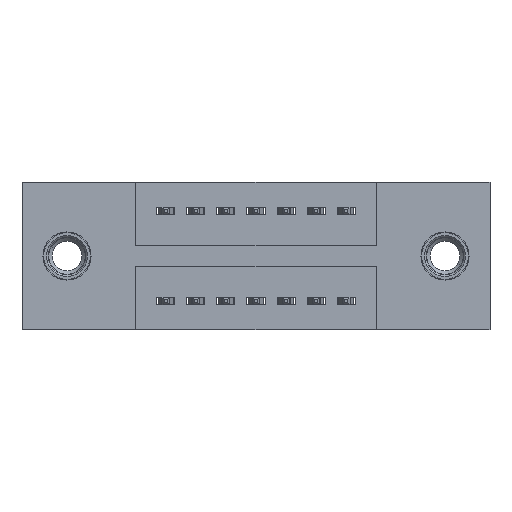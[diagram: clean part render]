
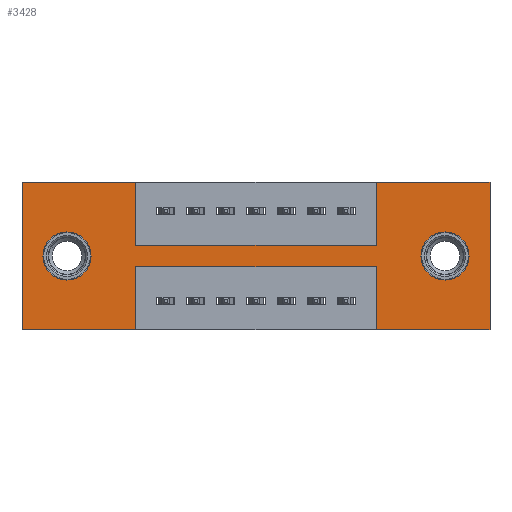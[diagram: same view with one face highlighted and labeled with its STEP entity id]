
A CAD part, front view. The second image highlights one B-rep face of the part: STEP entity #3428.
In plain terms, the highlighted planar face has unit normal (0, -1, 0).
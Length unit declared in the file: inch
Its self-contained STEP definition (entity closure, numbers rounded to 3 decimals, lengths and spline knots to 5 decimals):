
#21 = CARTESIAN_POINT ( 'NONE',  ( 1.1775, 0., -0.21 ) ) ;
#37 = LINE ( 'NONE', #5412, #4712 ) ;
#137 = AXIS2_PLACEMENT_3D ( 'NONE', #9034, #8138, #1855 ) ;
#304 = CARTESIAN_POINT ( 'NONE',  ( 1.4055, 0., -0.325 ) ) ;
#337 = EDGE_CURVE ( 'NONE', #5619, #1112, #37, .T. ) ;
#703 = ORIENTED_EDGE ( 'NONE', *, *, #7558, .T. ) ;
#708 = EDGE_CURVE ( 'NONE', #3977, #9456, #5096, .T. ) ;
#747 = ORIENTED_EDGE ( 'NONE', *, *, #9672, .T. ) ;
#772 = DIRECTION ( 'NONE',  ( -1., 0., 0. ) ) ;
#847 = VERTEX_POINT ( 'NONE', #9888 ) ;
#853 = CARTESIAN_POINT ( 'NONE',  ( 0.1495, 0., -0.245 ) ) ;
#908 = ORIENTED_EDGE ( 'NONE', *, *, #8822, .F. ) ;
#981 = ORIENTED_EDGE ( 'NONE', *, *, #4934, .F. ) ;
#989 = EDGE_CURVE ( 'NONE', #1058, #3947, #5598, .T. ) ;
#1058 = VERTEX_POINT ( 'NONE', #7208 ) ;
#1087 = EDGE_CURVE ( 'NONE', #4952, #6280, #4231, .T. ) ;
#1112 = VERTEX_POINT ( 'NONE', #4107 ) ;
#1210 = CARTESIAN_POINT ( 'NONE',  ( 0.3775, 0., -0.28 ) ) ;
#1282 = DIRECTION ( 'NONE',  ( 0., 0., -1. ) ) ;
#1493 = ORIENTED_EDGE ( 'NONE', *, *, #1875, .F. ) ;
#1513 = DIRECTION ( 'NONE',  ( 0., 0., -1. ) ) ;
#1626 = CARTESIAN_POINT ( 'NONE',  ( 1.1775, 0., -0.49 ) ) ;
#1719 = VECTOR ( 'NONE', #6772, 39.37008 ) ;
#1808 = DIRECTION ( 'NONE',  ( 1., 0., 0. ) ) ;
#1855 = DIRECTION ( 'NONE',  ( 0., 0., -1. ) ) ;
#1875 = EDGE_CURVE ( 'NONE', #847, #4952, #6077, .T. ) ;
#1997 = DIRECTION ( 'NONE',  ( 0., 1., 0. ) ) ;
#2097 = CARTESIAN_POINT ( 'NONE',  ( 1.1775, 0., -0.21 ) ) ;
#2109 = VECTOR ( 'NONE', #772, 39.37008 ) ;
#2134 = CARTESIAN_POINT ( 'NONE',  ( 1.4055, 0., -0.245 ) ) ;
#2318 = LINE ( 'NONE', #7312, #7439 ) ;
#2437 = DIRECTION ( 'NONE',  ( -1., 0., 0. ) ) ;
#2461 = EDGE_CURVE ( 'NONE', #9456, #7937, #5810, .T. ) ;
#2532 = DIRECTION ( 'NONE',  ( 0., 0., 1. ) ) ;
#2781 = DIRECTION ( 'NONE',  ( 0., 0., 1. ) ) ;
#2905 = CARTESIAN_POINT ( 'NONE',  ( 0.1495, 0., -0.325 ) ) ;
#3004 = VERTEX_POINT ( 'NONE', #3969 ) ;
#3428 = ADVANCED_FACE ( 'NONE', ( #10253, #8640, #8649 ), #7069, .T. ) ;
#3559 = LINE ( 'NONE', #6745, #9177 ) ;
#3593 = VERTEX_POINT ( 'NONE', #5746 ) ;
#3770 = AXIS2_PLACEMENT_3D ( 'NONE', #853, #4056, #7134 ) ;
#3772 = CARTESIAN_POINT ( 'NONE',  ( 0., 0., 0. ) ) ;
#3821 = DIRECTION ( 'NONE',  ( 0., 0., -1. ) ) ;
#3862 = EDGE_LOOP ( 'NONE', ( #747, #5677 ) ) ;
#3917 = ORIENTED_EDGE ( 'NONE', *, *, #2461, .F. ) ;
#3918 = VECTOR ( 'NONE', #4582, 39.37008 ) ;
#3947 = VERTEX_POINT ( 'NONE', #2905 ) ;
#3969 = CARTESIAN_POINT ( 'NONE',  ( 1.1775, 0., 0. ) ) ;
#3977 = VERTEX_POINT ( 'NONE', #5399 ) ;
#4003 = EDGE_CURVE ( 'NONE', #3004, #847, #8522, .T. ) ;
#4014 = ORIENTED_EDGE ( 'NONE', *, *, #8997, .F. ) ;
#4056 = DIRECTION ( 'NONE',  ( 0., 1., 0. ) ) ;
#4107 = CARTESIAN_POINT ( 'NONE',  ( 0.3775, 0., -0.21 ) ) ;
#4170 = AXIS2_PLACEMENT_3D ( 'NONE', #2134, #7713, #1282 ) ;
#4183 = DIRECTION ( 'NONE',  ( -1., 0., 0. ) ) ;
#4184 = VECTOR ( 'NONE', #5045, 39.37008 ) ;
#4231 = LINE ( 'NONE', #5546, #2109 ) ;
#4523 = VECTOR ( 'NONE', #5766, 39.37008 ) ;
#4567 = VERTEX_POINT ( 'NONE', #9597 ) ;
#4582 = DIRECTION ( 'NONE',  ( 1., 0., 0. ) ) ;
#4712 = VECTOR ( 'NONE', #1513, 39.37008 ) ;
#4934 = EDGE_CURVE ( 'NONE', #3593, #4567, #9391, .T. ) ;
#4939 = CARTESIAN_POINT ( 'NONE',  ( 0., 0., -0.49 ) ) ;
#4944 = LINE ( 'NONE', #2097, #1719 ) ;
#4952 = VERTEX_POINT ( 'NONE', #5337 ) ;
#5045 = DIRECTION ( 'NONE',  ( 0., 0., -1. ) ) ;
#5096 = LINE ( 'NONE', #8062, #9454 ) ;
#5138 = AXIS2_PLACEMENT_3D ( 'NONE', #6761, #1997, #2781 ) ;
#5332 = CARTESIAN_POINT ( 'NONE',  ( 0.3775, 0., -0.28 ) ) ;
#5337 = CARTESIAN_POINT ( 'NONE',  ( 1.555, 0., -0.49 ) ) ;
#5399 = CARTESIAN_POINT ( 'NONE',  ( 1.1775, 0., -0.28 ) ) ;
#5412 = CARTESIAN_POINT ( 'NONE',  ( 0.3775, 0., -0.21 ) ) ;
#5446 = CARTESIAN_POINT ( 'NONE',  ( 0., 0., -0.49 ) ) ;
#5469 = ORIENTED_EDGE ( 'NONE', *, *, #8075, .F. ) ;
#5546 = CARTESIAN_POINT ( 'NONE',  ( 0., 0., -0.49 ) ) ;
#5598 = CIRCLE ( 'NONE', #5138, 0.08 ) ;
#5619 = VERTEX_POINT ( 'NONE', #7851 ) ;
#5630 = CARTESIAN_POINT ( 'NONE',  ( 1.4055, 0., -0.165 ) ) ;
#5677 = ORIENTED_EDGE ( 'NONE', *, *, #9296, .T. ) ;
#5746 = CARTESIAN_POINT ( 'NONE',  ( 0., 0., -0.49 ) ) ;
#5766 = DIRECTION ( 'NONE',  ( 0., 0., 1. ) ) ;
#5810 = LINE ( 'NONE', #1210, #4184 ) ;
#5844 = CIRCLE ( 'NONE', #3770, 0.08 ) ;
#5938 = LINE ( 'NONE', #4939, #7951 ) ;
#6068 = AXIS2_PLACEMENT_3D ( 'NONE', #5446, #7787, #3821 ) ;
#6077 = LINE ( 'NONE', #9421, #10173 ) ;
#6165 = CIRCLE ( 'NONE', #137, 0.08 ) ;
#6280 = VERTEX_POINT ( 'NONE', #1626 ) ;
#6313 = VERTEX_POINT ( 'NONE', #5630 ) ;
#6340 = ORIENTED_EDGE ( 'NONE', *, *, #8435, .F. ) ;
#6370 = ORIENTED_EDGE ( 'NONE', *, *, #337, .F. ) ;
#6745 = CARTESIAN_POINT ( 'NONE',  ( 0., 0., 0. ) ) ;
#6761 = CARTESIAN_POINT ( 'NONE',  ( 0.1495, 0., -0.245 ) ) ;
#6772 = DIRECTION ( 'NONE',  ( 0., 0., 1. ) ) ;
#7069 = PLANE ( 'NONE',  #6068 ) ;
#7088 = DIRECTION ( 'NONE',  ( 1., 0., 0. ) ) ;
#7134 = DIRECTION ( 'NONE',  ( 0., 0., 1. ) ) ;
#7208 = CARTESIAN_POINT ( 'NONE',  ( 0.1495, 0., -0.165 ) ) ;
#7286 = CARTESIAN_POINT ( 'NONE',  ( 0.3775, 0., -0.21 ) ) ;
#7312 = CARTESIAN_POINT ( 'NONE',  ( 1.1775, 0., -0.28 ) ) ;
#7439 = VECTOR ( 'NONE', #2532, 39.37008 ) ;
#7454 = EDGE_LOOP ( 'NONE', ( #8608, #703 ) ) ;
#7558 = EDGE_CURVE ( 'NONE', #3947, #1058, #5844, .T. ) ;
#7581 = ORIENTED_EDGE ( 'NONE', *, *, #1087, .F. ) ;
#7713 = DIRECTION ( 'NONE',  ( 0., 1., 0. ) ) ;
#7787 = DIRECTION ( 'NONE',  ( 0., -1., 0. ) ) ;
#7851 = CARTESIAN_POINT ( 'NONE',  ( 0.3775, 0., 0. ) ) ;
#7937 = VERTEX_POINT ( 'NONE', #8999 ) ;
#7951 = VECTOR ( 'NONE', #4183, 39.37008 ) ;
#7980 = VERTEX_POINT ( 'NONE', #304 ) ;
#8062 = CARTESIAN_POINT ( 'NONE',  ( 0.3775, 0., -0.28 ) ) ;
#8075 = EDGE_CURVE ( 'NONE', #9611, #3004, #4944, .T. ) ;
#8138 = DIRECTION ( 'NONE',  ( 0., 1., 0. ) ) ;
#8206 = ORIENTED_EDGE ( 'NONE', *, *, #708, .F. ) ;
#8337 = ORIENTED_EDGE ( 'NONE', *, *, #8427, .F. ) ;
#8427 = EDGE_CURVE ( 'NONE', #1112, #9611, #9062, .T. ) ;
#8435 = EDGE_CURVE ( 'NONE', #7937, #3593, #5938, .T. ) ;
#8522 = LINE ( 'NONE', #3772, #3918 ) ;
#8608 = ORIENTED_EDGE ( 'NONE', *, *, #989, .T. ) ;
#8640 = FACE_BOUND ( 'NONE', #7454, .T. ) ;
#8649 = FACE_OUTER_BOUND ( 'NONE', #8691, .T. ) ;
#8664 = DIRECTION ( 'NONE',  ( 0., 0., -1. ) ) ;
#8691 = EDGE_LOOP ( 'NONE', ( #5469, #8337, #6370, #4014, #981, #6340, #3917, #8206, #908, #7581, #1493, #9082 ) ) ;
#8822 = EDGE_CURVE ( 'NONE', #6280, #3977, #2318, .T. ) ;
#8928 = CARTESIAN_POINT ( 'NONE',  ( 0., 0., 0. ) ) ;
#8997 = EDGE_CURVE ( 'NONE', #4567, #5619, #3559, .T. ) ;
#8999 = CARTESIAN_POINT ( 'NONE',  ( 0.3775, 0., -0.49 ) ) ;
#9034 = CARTESIAN_POINT ( 'NONE',  ( 1.4055, 0., -0.245 ) ) ;
#9062 = LINE ( 'NONE', #7286, #10040 ) ;
#9082 = ORIENTED_EDGE ( 'NONE', *, *, #4003, .F. ) ;
#9177 = VECTOR ( 'NONE', #7088, 39.37008 ) ;
#9296 = EDGE_CURVE ( 'NONE', #7980, #6313, #6165, .T. ) ;
#9391 = LINE ( 'NONE', #8928, #4523 ) ;
#9421 = CARTESIAN_POINT ( 'NONE',  ( 1.555, 0., 0. ) ) ;
#9454 = VECTOR ( 'NONE', #2437, 39.37008 ) ;
#9456 = VERTEX_POINT ( 'NONE', #5332 ) ;
#9597 = CARTESIAN_POINT ( 'NONE',  ( 0., 0., 0. ) ) ;
#9611 = VERTEX_POINT ( 'NONE', #21 ) ;
#9672 = EDGE_CURVE ( 'NONE', #6313, #7980, #10135, .T. ) ;
#9888 = CARTESIAN_POINT ( 'NONE',  ( 1.555, 0., 0. ) ) ;
#10040 = VECTOR ( 'NONE', #1808, 39.37008 ) ;
#10135 = CIRCLE ( 'NONE', #4170, 0.08 ) ;
#10173 = VECTOR ( 'NONE', #8664, 39.37008 ) ;
#10253 = FACE_BOUND ( 'NONE', #3862, .T. ) ;
